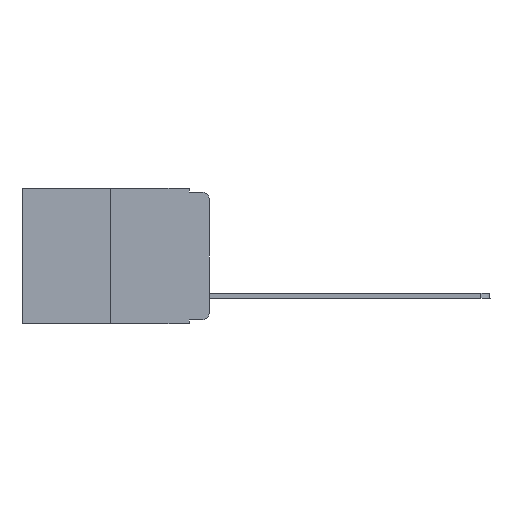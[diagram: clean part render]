
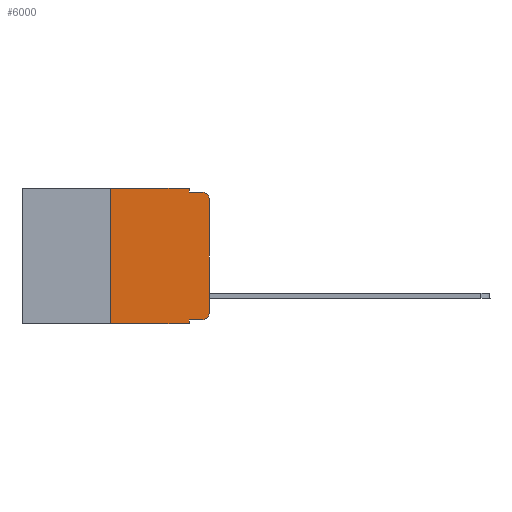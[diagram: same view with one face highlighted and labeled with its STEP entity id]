
A CAD part, left-side view. The second image highlights one B-rep face of the part: STEP entity #6000.
In plain terms, the highlighted planar face has unit normal (-1, 0, 0).
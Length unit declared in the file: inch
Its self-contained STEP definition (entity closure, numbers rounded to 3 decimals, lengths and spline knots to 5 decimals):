
#251 = EDGE_CURVE ( 'NONE', #12637, #7798, #4198, .T. ) ;
#376 = EDGE_CURVE ( 'NONE', #2491, #8314, #1217, .T. ) ;
#703 = DIRECTION ( 'NONE',  ( -1., 0., 0. ) ) ;
#966 = DIRECTION ( 'NONE',  ( -1., 0., 0. ) ) ;
#1217 = LINE ( 'NONE', #8578, #10512 ) ;
#1272 = DIRECTION ( 'NONE',  ( 0., -1., 0. ) ) ;
#1357 = VERTEX_POINT ( 'NONE', #11059 ) ;
#1558 = EDGE_CURVE ( 'NONE', #10518, #4326, #7296, .T. ) ;
#1944 = EDGE_CURVE ( 'NONE', #9045, #8314, #10474, .T. ) ;
#2107 = ORIENTED_EDGE ( 'NONE', *, *, #10375, .T. ) ;
#2221 = DIRECTION ( 'NONE',  ( 0., -1., 0. ) ) ;
#2347 = EDGE_CURVE ( 'NONE', #2491, #1357, #10950, .T. ) ;
#2352 = VECTOR ( 'NONE', #9155, 39.37008 ) ;
#2433 = VECTOR ( 'NONE', #11803, 39.37008 ) ;
#2491 = VERTEX_POINT ( 'NONE', #11994 ) ;
#2804 = LINE ( 'NONE', #9985, #2975 ) ;
#2807 = DIRECTION ( 'NONE',  ( 0., 0., -1. ) ) ;
#2896 = AXIS2_PLACEMENT_3D ( 'NONE', #4181, #703, #5480 ) ;
#2959 = ORIENTED_EDGE ( 'NONE', *, *, #8391, .F. ) ;
#2975 = VECTOR ( 'NONE', #8907, 39.37008 ) ;
#3184 = CARTESIAN_POINT ( 'NONE',  ( 0., 0.02, -0.313 ) ) ;
#3312 = DIRECTION ( 'NONE',  ( 0., 0., 1. ) ) ;
#3341 = LINE ( 'NONE', #8450, #7760 ) ;
#3504 = VECTOR ( 'NONE', #3312, 39.37008 ) ;
#3543 = CARTESIAN_POINT ( 'NONE',  ( 0., 0.051, 0. ) ) ;
#3724 = ORIENTED_EDGE ( 'NONE', *, *, #2347, .F. ) ;
#3963 = ORIENTED_EDGE ( 'NONE', *, *, #1558, .T. ) ;
#4065 = CARTESIAN_POINT ( 'NONE',  ( 0., 0.051, -0.333 ) ) ;
#4181 = CARTESIAN_POINT ( 'NONE',  ( 0., 0.02, -0.03 ) ) ;
#4198 = CIRCLE ( 'NONE', #8683, 0.02 ) ;
#4227 = EDGE_CURVE ( 'NONE', #9045, #12637, #3341, .T. ) ;
#4326 = VERTEX_POINT ( 'NONE', #5002 ) ;
#4391 = CARTESIAN_POINT ( 'NONE',  ( 0., 0.25, 0. ) ) ;
#4483 = CARTESIAN_POINT ( 'NONE',  ( 0., 0.473, 0. ) ) ;
#4643 = VERTEX_POINT ( 'NONE', #3543 ) ;
#4774 = FACE_OUTER_BOUND ( 'NONE', #12601, .T. ) ;
#4775 = ORIENTED_EDGE ( 'NONE', *, *, #7643, .F. ) ;
#5002 = CARTESIAN_POINT ( 'NONE',  ( 0., 0.02, -0.01 ) ) ;
#5480 = DIRECTION ( 'NONE',  ( 0., 0., -1. ) ) ;
#5809 = DIRECTION ( 'NONE',  ( 0., -1., 0. ) ) ;
#5869 = PLANE ( 'NONE',  #5896 ) ;
#5896 = AXIS2_PLACEMENT_3D ( 'NONE', #6785, #12277, #6875 ) ;
#6000 = ADVANCED_FACE ( 'NONE', ( #4774 ), #5869, .F. ) ;
#6340 = EDGE_CURVE ( 'NONE', #4643, #7526, #2804, .T. ) ;
#6727 = ORIENTED_EDGE ( 'NONE', *, *, #251, .T. ) ;
#6785 = CARTESIAN_POINT ( 'NONE',  ( 0., 0.473, 0. ) ) ;
#6875 = DIRECTION ( 'NONE',  ( 0., 0., -1. ) ) ;
#7296 = CIRCLE ( 'NONE', #2896, 0.02 ) ;
#7526 = VERTEX_POINT ( 'NONE', #9758 ) ;
#7643 = EDGE_CURVE ( 'NONE', #1357, #4643, #11188, .T. ) ;
#7760 = VECTOR ( 'NONE', #2221, 39.37008 ) ;
#7798 = VERTEX_POINT ( 'NONE', #12279 ) ;
#7972 = CARTESIAN_POINT ( 'NONE',  ( 0., 0.02, -0.333 ) ) ;
#8146 = CARTESIAN_POINT ( 'NONE',  ( 0., 0.051, 0. ) ) ;
#8294 = ORIENTED_EDGE ( 'NONE', *, *, #6340, .F. ) ;
#8314 = VERTEX_POINT ( 'NONE', #9742 ) ;
#8384 = ORIENTED_EDGE ( 'NONE', *, *, #1944, .F. ) ;
#8391 = EDGE_CURVE ( 'NONE', #7526, #4326, #8819, .T. ) ;
#8450 = CARTESIAN_POINT ( 'NONE',  ( 0., 0.051, -0.333 ) ) ;
#8552 = CARTESIAN_POINT ( 'NONE',  ( 0., 0., 0. ) ) ;
#8578 = CARTESIAN_POINT ( 'NONE',  ( 0., 0.473, -0.343 ) ) ;
#8679 = ORIENTED_EDGE ( 'NONE', *, *, #4227, .T. ) ;
#8683 = AXIS2_PLACEMENT_3D ( 'NONE', #3184, #966, #2807 ) ;
#8814 = CARTESIAN_POINT ( 'NONE',  ( 0., 0., -0.03 ) ) ;
#8819 = LINE ( 'NONE', #12307, #9488 ) ;
#8907 = DIRECTION ( 'NONE',  ( 0., 0., -1. ) ) ;
#9045 = VERTEX_POINT ( 'NONE', #4065 ) ;
#9155 = DIRECTION ( 'NONE',  ( 0., 0., -1. ) ) ;
#9333 = ORIENTED_EDGE ( 'NONE', *, *, #376, .T. ) ;
#9488 = VECTOR ( 'NONE', #5809, 39.37008 ) ;
#9742 = CARTESIAN_POINT ( 'NONE',  ( 0., 0.051, -0.343 ) ) ;
#9758 = CARTESIAN_POINT ( 'NONE',  ( 0., 0.051, -0.01 ) ) ;
#9985 = CARTESIAN_POINT ( 'NONE',  ( 0., 0.051, 0. ) ) ;
#10375 = EDGE_CURVE ( 'NONE', #7798, #10518, #11386, .T. ) ;
#10474 = LINE ( 'NONE', #8146, #2352 ) ;
#10512 = VECTOR ( 'NONE', #10724, 39.37008 ) ;
#10518 = VERTEX_POINT ( 'NONE', #8814 ) ;
#10724 = DIRECTION ( 'NONE',  ( 0., -1., 0. ) ) ;
#10950 = LINE ( 'NONE', #4391, #3504 ) ;
#11059 = CARTESIAN_POINT ( 'NONE',  ( 0., 0.25, 0. ) ) ;
#11188 = LINE ( 'NONE', #4483, #13319 ) ;
#11386 = LINE ( 'NONE', #8552, #2433 ) ;
#11803 = DIRECTION ( 'NONE',  ( 0., 0., 1. ) ) ;
#11994 = CARTESIAN_POINT ( 'NONE',  ( 0., 0.25, -0.343 ) ) ;
#12277 = DIRECTION ( 'NONE',  ( 1., 0., 0. ) ) ;
#12279 = CARTESIAN_POINT ( 'NONE',  ( 0., 0., -0.313 ) ) ;
#12307 = CARTESIAN_POINT ( 'NONE',  ( 0., 0.051, -0.01 ) ) ;
#12601 = EDGE_LOOP ( 'NONE', ( #2107, #3963, #2959, #8294, #4775, #3724, #9333, #8384, #8679, #6727 ) ) ;
#12637 = VERTEX_POINT ( 'NONE', #7972 ) ;
#13319 = VECTOR ( 'NONE', #1272, 39.37008 ) ;
